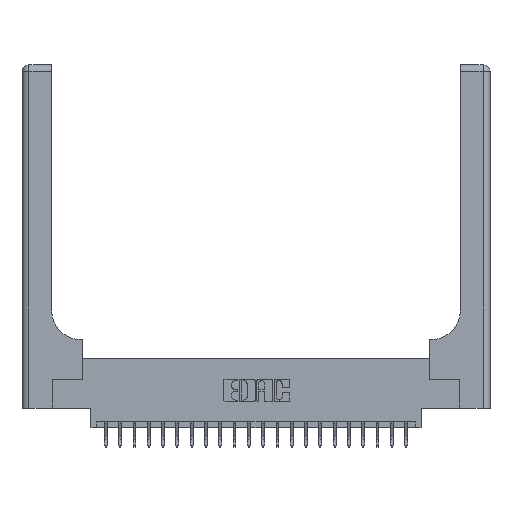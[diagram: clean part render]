
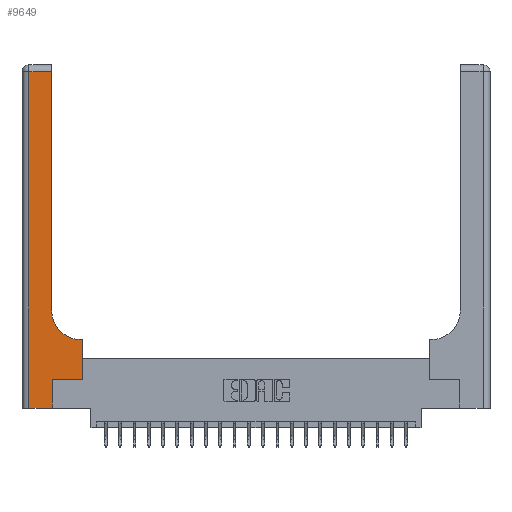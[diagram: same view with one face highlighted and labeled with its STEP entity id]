
A CAD part, top view. The second image highlights one B-rep face of the part: STEP entity #9649.
In plain terms, the highlighted planar face has unit normal (0, 0, 1).
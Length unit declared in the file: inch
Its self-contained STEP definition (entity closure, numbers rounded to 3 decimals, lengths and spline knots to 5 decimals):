
#105 = DIRECTION ( 'NONE',  ( -1., 0., 0. ) ) ;
#122 = DIRECTION ( 'NONE',  ( 1., 0., 0. ) ) ;
#342 = VERTEX_POINT ( 'NONE', #11766 ) ;
#486 = ORIENTED_EDGE ( 'NONE', *, *, #15234, .T. ) ;
#1085 = CARTESIAN_POINT ( 'NONE',  ( 0.265, 0.25, 0.37 ) ) ;
#1695 = VERTEX_POINT ( 'NONE', #2526 ) ;
#1752 = LINE ( 'NONE', #10412, #5876 ) ;
#2037 = CARTESIAN_POINT ( 'NONE',  ( 0.528, 0.6, 0.37 ) ) ;
#2053 = ORIENTED_EDGE ( 'NONE', *, *, #17221, .T. ) ;
#2109 = CARTESIAN_POINT ( 'NONE',  ( 0.528, 0.25, 0.37 ) ) ;
#2122 = CARTESIAN_POINT ( 'NONE',  ( 0.528, 0.25, 0.37 ) ) ;
#2415 = VECTOR ( 'NONE', #18304, 39.37008 ) ;
#2526 = CARTESIAN_POINT ( 'NONE',  ( 0.26, 2.94, 0.37 ) ) ;
#3966 = VERTEX_POINT ( 'NONE', #20691 ) ;
#4122 = EDGE_CURVE ( 'NONE', #1695, #6568, #5847, .T. ) ;
#4277 = ORIENTED_EDGE ( 'NONE', *, *, #21203, .T. ) ;
#4455 = CARTESIAN_POINT ( 'NONE',  ( 0.26, 0.85, 0.37 ) ) ;
#4466 = DIRECTION ( 'NONE',  ( -1., 0., 0. ) ) ;
#4894 = ORIENTED_EDGE ( 'NONE', *, *, #8338, .T. ) ;
#5141 = VECTOR ( 'NONE', #15110, 39.37008 ) ;
#5847 = LINE ( 'NONE', #15819, #10507 ) ;
#5876 = VECTOR ( 'NONE', #19095, 39.37008 ) ;
#5981 = LINE ( 'NONE', #2109, #14706 ) ;
#6568 = VERTEX_POINT ( 'NONE', #9090 ) ;
#6736 = EDGE_CURVE ( 'NONE', #21007, #3966, #20981, .T. ) ;
#7281 = FACE_OUTER_BOUND ( 'NONE', #16176, .T. ) ;
#8318 = ORIENTED_EDGE ( 'NONE', *, *, #6736, .T. ) ;
#8338 = EDGE_CURVE ( 'NONE', #11956, #21007, #12515, .T. ) ;
#8460 = EDGE_CURVE ( 'NONE', #3966, #16619, #19608, .T. ) ;
#8707 = ORIENTED_EDGE ( 'NONE', *, *, #4122, .T. ) ;
#8927 = VECTOR ( 'NONE', #4466, 39.37008 ) ;
#9090 = CARTESIAN_POINT ( 'NONE',  ( 0.06, 2.94, 0.37 ) ) ;
#9571 = EDGE_CURVE ( 'NONE', #21981, #342, #13548, .T. ) ;
#9574 = DIRECTION ( 'NONE',  ( 1., 0., 0. ) ) ;
#9649 = ADVANCED_FACE ( 'NONE', ( #7281 ), #16843, .F. ) ;
#9895 = CARTESIAN_POINT ( 'NONE',  ( 0., 3., 0.37 ) ) ;
#10203 = ORIENTED_EDGE ( 'NONE', *, *, #20140, .T. ) ;
#10412 = CARTESIAN_POINT ( 'NONE',  ( 0.06, 3., 0.37 ) ) ;
#10507 = VECTOR ( 'NONE', #105, 39.37008 ) ;
#10657 = DIRECTION ( 'NONE',  ( 0., 0., -1. ) ) ;
#10847 = DIRECTION ( 'NONE',  ( 0., 1., 0. ) ) ;
#11299 = CARTESIAN_POINT ( 'NONE',  ( 0., 0., 0.37 ) ) ;
#11639 = DIRECTION ( 'NONE',  ( -1., 0., 0. ) ) ;
#11766 = CARTESIAN_POINT ( 'NONE',  ( 0.51, 0.6, 0.37 ) ) ;
#11956 = VERTEX_POINT ( 'NONE', #16933 ) ;
#12515 = LINE ( 'NONE', #11299, #21211 ) ;
#13548 = LINE ( 'NONE', #16614, #8927 ) ;
#14558 = CARTESIAN_POINT ( 'NONE',  ( 0.26, 3., 0.37 ) ) ;
#14706 = VECTOR ( 'NONE', #10847, 39.37008 ) ;
#15043 = AXIS2_PLACEMENT_3D ( 'NONE', #9895, #22047, #11639 ) ;
#15110 = DIRECTION ( 'NONE',  ( 1., 0., 0. ) ) ;
#15126 = VERTEX_POINT ( 'NONE', #4455 ) ;
#15234 = EDGE_CURVE ( 'NONE', #6568, #11956, #1752, .T. ) ;
#15819 = CARTESIAN_POINT ( 'NONE',  ( 0., 2.94, 0.37 ) ) ;
#15942 = LINE ( 'NONE', #14558, #21082 ) ;
#16176 = EDGE_LOOP ( 'NONE', ( #2053, #8707, #486, #4894, #8318, #16461, #10203, #18028, #4277 ) ) ;
#16317 = DIRECTION ( 'NONE',  ( 0., 1., 0. ) ) ;
#16461 = ORIENTED_EDGE ( 'NONE', *, *, #8460, .T. ) ;
#16558 = CARTESIAN_POINT ( 'NONE',  ( 0.265, 0., 0.37 ) ) ;
#16614 = CARTESIAN_POINT ( 'NONE',  ( 0.26, 0.6, 0.37 ) ) ;
#16619 = VERTEX_POINT ( 'NONE', #2122 ) ;
#16843 = PLANE ( 'NONE',  #15043 ) ;
#16933 = CARTESIAN_POINT ( 'NONE',  ( 0.06, 0., 0.37 ) ) ;
#17221 = EDGE_CURVE ( 'NONE', #15126, #1695, #15942, .T. ) ;
#18028 = ORIENTED_EDGE ( 'NONE', *, *, #9571, .T. ) ;
#18304 = DIRECTION ( 'NONE',  ( 0., 1., 0. ) ) ;
#19095 = DIRECTION ( 'NONE',  ( 0., -1., 0. ) ) ;
#19608 = LINE ( 'NONE', #1085, #5141 ) ;
#20140 = EDGE_CURVE ( 'NONE', #16619, #21981, #5981, .T. ) ;
#20480 = CARTESIAN_POINT ( 'NONE',  ( 0.265, 0., 0.37 ) ) ;
#20691 = CARTESIAN_POINT ( 'NONE',  ( 0.265, 0.25, 0.37 ) ) ;
#20720 = AXIS2_PLACEMENT_3D ( 'NONE', #21056, #10657, #122 ) ;
#20981 = LINE ( 'NONE', #16558, #2415 ) ;
#21007 = VERTEX_POINT ( 'NONE', #20480 ) ;
#21056 = CARTESIAN_POINT ( 'NONE',  ( 0.51, 0.85, 0.37 ) ) ;
#21082 = VECTOR ( 'NONE', #16317, 39.37008 ) ;
#21177 = CIRCLE ( 'NONE', #20720, 0.25 ) ;
#21203 = EDGE_CURVE ( 'NONE', #342, #15126, #21177, .T. ) ;
#21211 = VECTOR ( 'NONE', #9574, 39.37008 ) ;
#21981 = VERTEX_POINT ( 'NONE', #2037 ) ;
#22047 = DIRECTION ( 'NONE',  ( 0., 0., -1. ) ) ;
